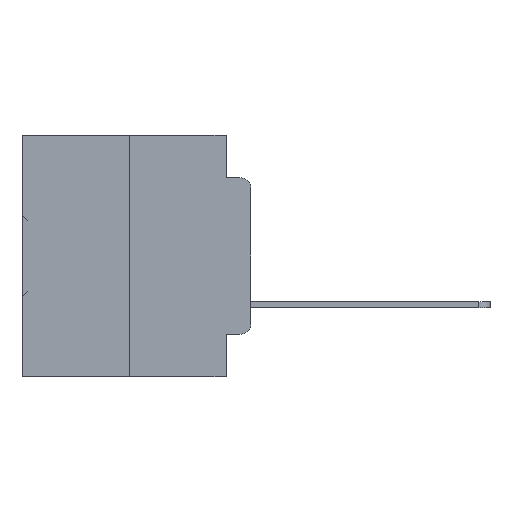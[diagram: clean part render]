
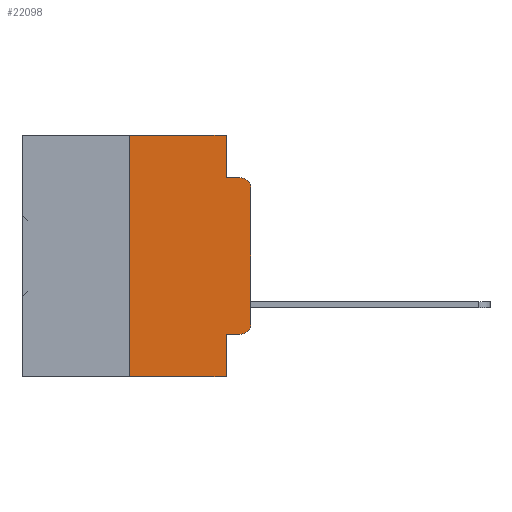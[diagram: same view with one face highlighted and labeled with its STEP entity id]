
A CAD part, left-side view. The second image highlights one B-rep face of the part: STEP entity #22098.
In plain terms, the highlighted planar face has unit normal (-1, 0, 0).
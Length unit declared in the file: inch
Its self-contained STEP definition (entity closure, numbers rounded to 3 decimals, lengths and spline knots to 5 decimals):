
#190 = EDGE_CURVE ( 'NONE', #28526, #2800, #22526, .T. ) ;
#1309 = ORIENTED_EDGE ( 'NONE', *, *, #17301, .F. ) ;
#1520 = EDGE_LOOP ( 'NONE', ( #13971, #7276, #5223, #6282, #2803, #1309, #17757, #5846, #2645, #7535 ) ) ;
#1919 = CARTESIAN_POINT ( 'NONE',  ( 0., 0.051, -0.5 ) ) ;
#2645 = ORIENTED_EDGE ( 'NONE', *, *, #20633, .T. ) ;
#2800 = VERTEX_POINT ( 'NONE', #20552 ) ;
#2803 = ORIENTED_EDGE ( 'NONE', *, *, #18850, .F. ) ;
#2876 = CARTESIAN_POINT ( 'NONE',  ( 0., 0.051, -0.0885 ) ) ;
#4226 = LINE ( 'NONE', #4953, #10714 ) ;
#4321 = EDGE_CURVE ( 'NONE', #7069, #36834, #31778, .T. ) ;
#4953 = CARTESIAN_POINT ( 'NONE',  ( 0., 0.051, 0. ) ) ;
#5126 = LINE ( 'NONE', #9874, #27087 ) ;
#5223 = ORIENTED_EDGE ( 'NONE', *, *, #38459, .F. ) ;
#5823 = EDGE_CURVE ( 'NONE', #32919, #36834, #36574, .T. ) ;
#5846 = ORIENTED_EDGE ( 'NONE', *, *, #5823, .F. ) ;
#6282 = ORIENTED_EDGE ( 'NONE', *, *, #7821, .F. ) ;
#6633 = VECTOR ( 'NONE', #27211, 39.37008 ) ;
#7069 = VERTEX_POINT ( 'NONE', #19755 ) ;
#7276 = ORIENTED_EDGE ( 'NONE', *, *, #31808, .T. ) ;
#7535 = ORIENTED_EDGE ( 'NONE', *, *, #31301, .T. ) ;
#7777 = PLANE ( 'NONE',  #7809 ) ;
#7809 = AXIS2_PLACEMENT_3D ( 'NONE', #22840, #31352, #14156 ) ;
#7821 = EDGE_CURVE ( 'NONE', #16278, #35824, #4226, .T. ) ;
#9088 = DIRECTION ( 'NONE',  ( -1., 0., 0. ) ) ;
#9874 = CARTESIAN_POINT ( 'NONE',  ( 0., 0.051, -0.4115 ) ) ;
#10047 = CARTESIAN_POINT ( 'NONE',  ( 0., 0.25, 0. ) ) ;
#10714 = VECTOR ( 'NONE', #14262, 39.37008 ) ;
#13018 = DIRECTION ( 'NONE',  ( 0., -1., 0. ) ) ;
#13702 = VECTOR ( 'NONE', #35083, 39.37008 ) ;
#13971 = ORIENTED_EDGE ( 'NONE', *, *, #190, .T. ) ;
#14156 = DIRECTION ( 'NONE',  ( 0., 0., -1. ) ) ;
#14254 = DIRECTION ( 'NONE',  ( 0., -1., 0. ) ) ;
#14262 = DIRECTION ( 'NONE',  ( 0., 0., -1. ) ) ;
#14953 = VECTOR ( 'NONE', #35168, 39.37008 ) ;
#15053 = VERTEX_POINT ( 'NONE', #38349 ) ;
#15509 = CARTESIAN_POINT ( 'NONE',  ( 0., 0.02, -0.3915 ) ) ;
#16278 = VERTEX_POINT ( 'NONE', #21844 ) ;
#16578 = VECTOR ( 'NONE', #14254, 39.37008 ) ;
#17301 = EDGE_CURVE ( 'NONE', #7069, #17532, #22695, .T. ) ;
#17532 = VERTEX_POINT ( 'NONE', #10047 ) ;
#17757 = ORIENTED_EDGE ( 'NONE', *, *, #4321, .T. ) ;
#18469 = DIRECTION ( 'NONE',  ( 0., 0., -1. ) ) ;
#18850 = EDGE_CURVE ( 'NONE', #17532, #16278, #31021, .T. ) ;
#19755 = CARTESIAN_POINT ( 'NONE',  ( 0., 0.25, -0.5 ) ) ;
#20008 = DIRECTION ( 'NONE',  ( 0., -1., 0. ) ) ;
#20016 = DIRECTION ( 'NONE',  ( 0., 0., 1. ) ) ;
#20552 = CARTESIAN_POINT ( 'NONE',  ( 0., 0., -0.1085 ) ) ;
#20633 = EDGE_CURVE ( 'NONE', #32919, #15053, #5126, .T. ) ;
#21844 = CARTESIAN_POINT ( 'NONE',  ( 0., 0.051, 0. ) ) ;
#22098 = ADVANCED_FACE ( 'NONE', ( #24837 ), #7777, .F. ) ;
#22526 = LINE ( 'NONE', #27473, #27414 ) ;
#22695 = LINE ( 'NONE', #32311, #14953 ) ;
#22840 = CARTESIAN_POINT ( 'NONE',  ( 0., 0.473, 0. ) ) ;
#23239 = CARTESIAN_POINT ( 'NONE',  ( 0., 0.051, -0.4115 ) ) ;
#24272 = CARTESIAN_POINT ( 'NONE',  ( 0., 0.051, -0.0885 ) ) ;
#24837 = FACE_OUTER_BOUND ( 'NONE', #1520, .T. ) ;
#26769 = CARTESIAN_POINT ( 'NONE',  ( 0., 0.02, -0.1085 ) ) ;
#26784 = CARTESIAN_POINT ( 'NONE',  ( 0., 0., -0.3915 ) ) ;
#27087 = VECTOR ( 'NONE', #13018, 39.37008 ) ;
#27211 = DIRECTION ( 'NONE',  ( 0., -1., 0. ) ) ;
#27414 = VECTOR ( 'NONE', #20016, 39.37008 ) ;
#27473 = CARTESIAN_POINT ( 'NONE',  ( 0., 0., 0. ) ) ;
#28526 = VERTEX_POINT ( 'NONE', #26784 ) ;
#28627 = CARTESIAN_POINT ( 'NONE',  ( 0., 0.473, -0.5 ) ) ;
#29592 = DIRECTION ( 'NONE',  ( 0., 0., -1. ) ) ;
#30182 = LINE ( 'NONE', #24272, #6633 ) ;
#31021 = LINE ( 'NONE', #34140, #37648 ) ;
#31301 = EDGE_CURVE ( 'NONE', #15053, #28526, #35443, .T. ) ;
#31352 = DIRECTION ( 'NONE',  ( 1., 0., 0. ) ) ;
#31778 = LINE ( 'NONE', #28627, #16578 ) ;
#31808 = EDGE_CURVE ( 'NONE', #2800, #38311, #34527, .T. ) ;
#32140 = CARTESIAN_POINT ( 'NONE',  ( 0., 0.02, -0.0885 ) ) ;
#32311 = CARTESIAN_POINT ( 'NONE',  ( 0., 0.25, 0. ) ) ;
#32919 = VERTEX_POINT ( 'NONE', #23239 ) ;
#33232 = AXIS2_PLACEMENT_3D ( 'NONE', #15509, #35506, #18469 ) ;
#34140 = CARTESIAN_POINT ( 'NONE',  ( 0., 0.473, 0. ) ) ;
#34527 = CIRCLE ( 'NONE', #36318, 0.02 ) ;
#35083 = DIRECTION ( 'NONE',  ( 0., 0., -1. ) ) ;
#35168 = DIRECTION ( 'NONE',  ( 0., 0., 1. ) ) ;
#35443 = CIRCLE ( 'NONE', #33232, 0.02 ) ;
#35506 = DIRECTION ( 'NONE',  ( -1., 0., 0. ) ) ;
#35824 = VERTEX_POINT ( 'NONE', #2876 ) ;
#36318 = AXIS2_PLACEMENT_3D ( 'NONE', #26769, #9088, #29592 ) ;
#36574 = LINE ( 'NONE', #37893, #13702 ) ;
#36834 = VERTEX_POINT ( 'NONE', #1919 ) ;
#37648 = VECTOR ( 'NONE', #20008, 39.37008 ) ;
#37893 = CARTESIAN_POINT ( 'NONE',  ( 0., 0.051, 0. ) ) ;
#38311 = VERTEX_POINT ( 'NONE', #32140 ) ;
#38349 = CARTESIAN_POINT ( 'NONE',  ( 0., 0.02, -0.4115 ) ) ;
#38459 = EDGE_CURVE ( 'NONE', #35824, #38311, #30182, .T. ) ;
